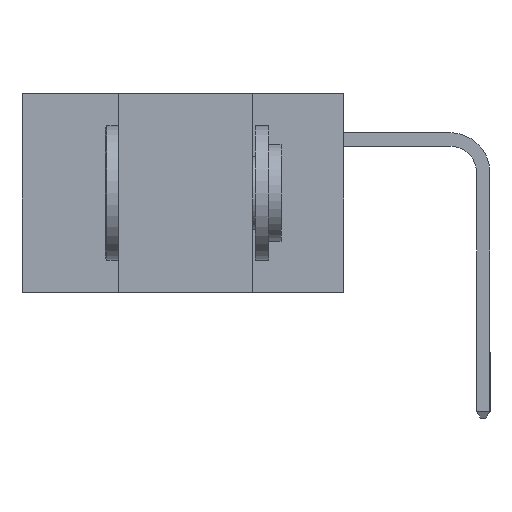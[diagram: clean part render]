
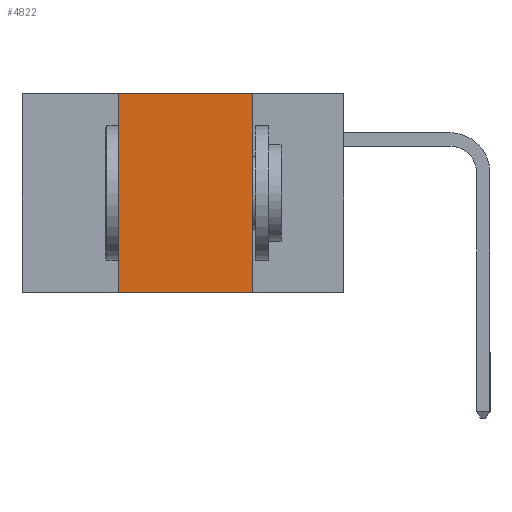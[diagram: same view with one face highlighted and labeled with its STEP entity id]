
A CAD part, left-side view. The second image highlights one B-rep face of the part: STEP entity #4822.
In plain terms, the highlighted planar face has unit normal (-1, 0, 0).
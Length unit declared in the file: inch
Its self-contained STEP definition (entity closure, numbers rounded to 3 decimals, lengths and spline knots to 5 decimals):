
#458 = ORIENTED_EDGE ( 'NONE', *, *, #9631, .T. ) ;
#628 = DIRECTION ( 'NONE',  ( 0., -1., 0. ) ) ;
#869 = LINE ( 'NONE', #7692, #8548 ) ;
#1039 = DIRECTION ( 'NONE',  ( 0., -1., 0. ) ) ;
#1161 = VECTOR ( 'NONE', #1039, 39.37008 ) ;
#1214 = ORIENTED_EDGE ( 'NONE', *, *, #8738, .F. ) ;
#1663 = VERTEX_POINT ( 'NONE', #7804 ) ;
#1701 = EDGE_CURVE ( 'NONE', #1663, #4772, #8466, .T. ) ;
#2078 = ORIENTED_EDGE ( 'NONE', *, *, #1701, .F. ) ;
#2258 = CARTESIAN_POINT ( 'NONE',  ( 0., 0.42, 0. ) ) ;
#2365 = CARTESIAN_POINT ( 'NONE',  ( 0., 0.6, 0. ) ) ;
#2409 = DIRECTION ( 'NONE',  ( 1., 0., 0. ) ) ;
#3274 = DIRECTION ( 'NONE',  ( 0., 0., -1. ) ) ;
#3378 = CARTESIAN_POINT ( 'NONE',  ( 0., 0.17, -0.37 ) ) ;
#3650 = VECTOR ( 'NONE', #3274, 39.37008 ) ;
#4689 = DIRECTION ( 'NONE',  ( 0., 0., 1. ) ) ;
#4772 = VERTEX_POINT ( 'NONE', #2258 ) ;
#4822 = ADVANCED_FACE ( 'NONE', ( #6488 ), #7878, .F. ) ;
#4957 = DIRECTION ( 'NONE',  ( 0., 0., -1. ) ) ;
#5030 = EDGE_LOOP ( 'NONE', ( #6489, #1214, #2078, #458 ) ) ;
#5447 = CARTESIAN_POINT ( 'NONE',  ( 0., 0.42, -0.37 ) ) ;
#5509 = LINE ( 'NONE', #3378, #3650 ) ;
#6488 = FACE_OUTER_BOUND ( 'NONE', #5030, .T. ) ;
#6489 = ORIENTED_EDGE ( 'NONE', *, *, #9629, .F. ) ;
#6950 = CARTESIAN_POINT ( 'NONE',  ( 0., 0.17, -0.37 ) ) ;
#7606 = AXIS2_PLACEMENT_3D ( 'NONE', #2365, #2409, #4957 ) ;
#7692 = CARTESIAN_POINT ( 'NONE',  ( 0., 0.6, 0. ) ) ;
#7804 = CARTESIAN_POINT ( 'NONE',  ( 0., 0.42, -0.37 ) ) ;
#7878 = PLANE ( 'NONE',  #7606 ) ;
#8030 = VECTOR ( 'NONE', #4689, 39.37008 ) ;
#8098 = LINE ( 'NONE', #8766, #1161 ) ;
#8466 = LINE ( 'NONE', #5447, #8030 ) ;
#8548 = VECTOR ( 'NONE', #628, 39.37008 ) ;
#8738 = EDGE_CURVE ( 'NONE', #4772, #8825, #869, .T. ) ;
#8766 = CARTESIAN_POINT ( 'NONE',  ( 0., 0.6, -0.37 ) ) ;
#8825 = VERTEX_POINT ( 'NONE', #9573 ) ;
#9092 = VERTEX_POINT ( 'NONE', #6950 ) ;
#9573 = CARTESIAN_POINT ( 'NONE',  ( 0., 0.17, 0. ) ) ;
#9629 = EDGE_CURVE ( 'NONE', #8825, #9092, #5509, .T. ) ;
#9631 = EDGE_CURVE ( 'NONE', #1663, #9092, #8098, .T. ) ;
